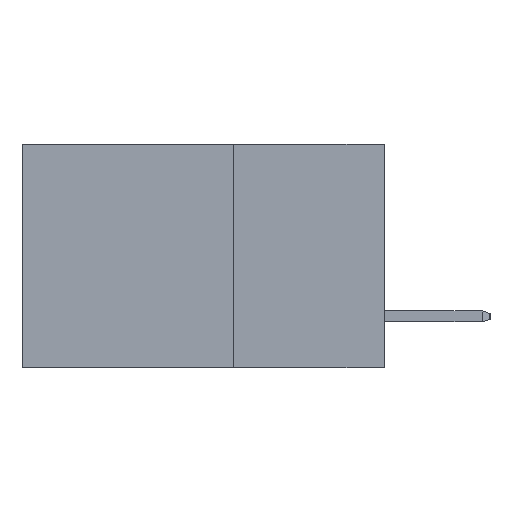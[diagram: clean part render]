
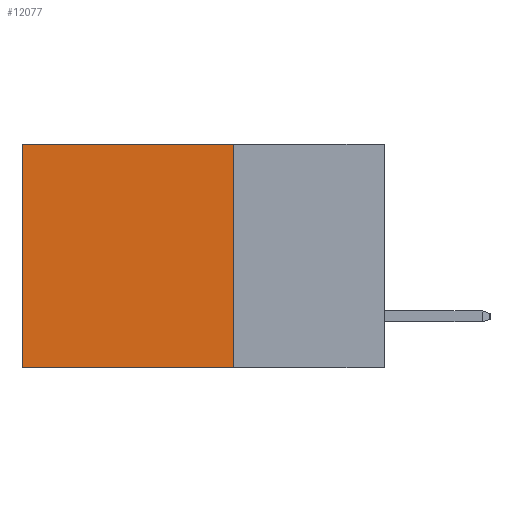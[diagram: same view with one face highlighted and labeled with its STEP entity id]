
A CAD part, left-side view. The second image highlights one B-rep face of the part: STEP entity #12077.
In plain terms, the highlighted planar face has unit normal (-1, 0, 0).
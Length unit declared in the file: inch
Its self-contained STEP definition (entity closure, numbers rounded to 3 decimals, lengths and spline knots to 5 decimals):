
#905 = LINE ( 'NONE', #3915, #18982 ) ;
#1104 = CARTESIAN_POINT ( 'NONE',  ( 0.298, 0.6, -0.37 ) ) ;
#2305 = DIRECTION ( 'NONE',  ( 0., 1., 0. ) ) ;
#3001 = LINE ( 'NONE', #4712, #15029 ) ;
#3915 = CARTESIAN_POINT ( 'NONE',  ( 0.298, 0.6, 0. ) ) ;
#4168 = PLANE ( 'NONE',  #23178 ) ;
#4283 = EDGE_CURVE ( 'NONE', #28091, #11177, #25601, .T. ) ;
#4319 = ORIENTED_EDGE ( 'NONE', *, *, #14581, .F. ) ;
#4605 = CARTESIAN_POINT ( 'NONE',  ( 0.298, 0.25, 0. ) ) ;
#4712 = CARTESIAN_POINT ( 'NONE',  ( 0.298, 0.25, -0.37 ) ) ;
#5706 = LINE ( 'NONE', #8523, #17705 ) ;
#6588 = DIRECTION ( 'NONE',  ( 1., 0., 0. ) ) ;
#8315 = CARTESIAN_POINT ( 'NONE',  ( 0.298, 0.25, 0. ) ) ;
#8523 = CARTESIAN_POINT ( 'NONE',  ( 0.298, 0.25, 0. ) ) ;
#11177 = VERTEX_POINT ( 'NONE', #17644 ) ;
#12077 = ADVANCED_FACE ( 'NONE', ( #16711 ), #4168, .F. ) ;
#12610 = EDGE_CURVE ( 'NONE', #11177, #26174, #905, .T. ) ;
#13466 = DIRECTION ( 'NONE',  ( 0., 0., -1. ) ) ;
#13603 = ORIENTED_EDGE ( 'NONE', *, *, #12610, .T. ) ;
#14177 = ORIENTED_EDGE ( 'NONE', *, *, #4283, .T. ) ;
#14581 = EDGE_CURVE ( 'NONE', #28091, #28755, #5706, .T. ) ;
#15029 = VECTOR ( 'NONE', #2305, 39.37008 ) ;
#15681 = EDGE_CURVE ( 'NONE', #28755, #26174, #3001, .T. ) ;
#16257 = ORIENTED_EDGE ( 'NONE', *, *, #15681, .F. ) ;
#16711 = FACE_OUTER_BOUND ( 'NONE', #26873, .T. ) ;
#17644 = CARTESIAN_POINT ( 'NONE',  ( 0.298, 0.6, 0. ) ) ;
#17705 = VECTOR ( 'NONE', #27434, 39.37008 ) ;
#18982 = VECTOR ( 'NONE', #13466, 39.37008 ) ;
#23178 = AXIS2_PLACEMENT_3D ( 'NONE', #27695, #6588, #23221 ) ;
#23221 = DIRECTION ( 'NONE',  ( 0., 0., -1. ) ) ;
#23920 = CARTESIAN_POINT ( 'NONE',  ( 0.298, 0.25, -0.37 ) ) ;
#25601 = LINE ( 'NONE', #8315, #26315 ) ;
#26174 = VERTEX_POINT ( 'NONE', #1104 ) ;
#26315 = VECTOR ( 'NONE', #27211, 39.37008 ) ;
#26873 = EDGE_LOOP ( 'NONE', ( #13603, #16257, #4319, #14177 ) ) ;
#27211 = DIRECTION ( 'NONE',  ( 0., 1., 0. ) ) ;
#27434 = DIRECTION ( 'NONE',  ( 0., 0., -1. ) ) ;
#27695 = CARTESIAN_POINT ( 'NONE',  ( 0.298, 0.25, 0. ) ) ;
#28091 = VERTEX_POINT ( 'NONE', #4605 ) ;
#28755 = VERTEX_POINT ( 'NONE', #23920 ) ;
